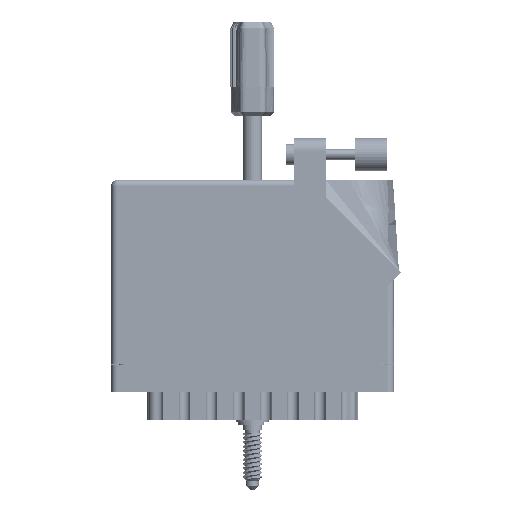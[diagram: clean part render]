
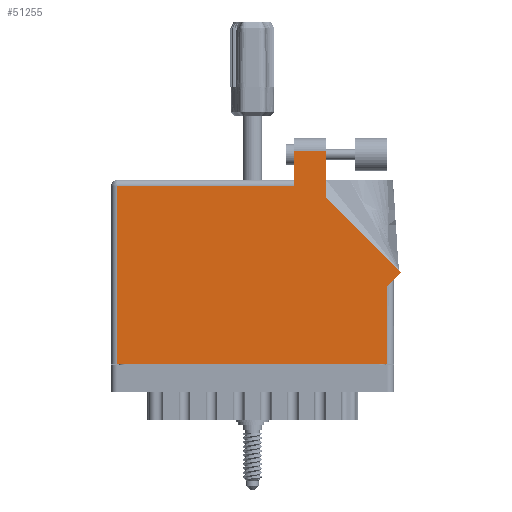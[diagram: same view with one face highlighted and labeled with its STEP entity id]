
A CAD part, front view. The second image highlights one B-rep face of the part: STEP entity #51255.
In plain terms, the highlighted face is planar.
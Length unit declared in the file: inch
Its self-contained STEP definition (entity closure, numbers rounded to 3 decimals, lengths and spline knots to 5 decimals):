
#1090 = CARTESIAN_POINT ( 'NONE',  ( 2.78871, 0.88571, 0. ) ) ;
#1462 = EDGE_LOOP ( 'NONE', ( #5592, #52478, #9378, #9748, #86802, #61947, #65933, #56642, #20698 ) ) ;
#2044 = VERTEX_POINT ( 'NONE', #49506 ) ;
#2688 = VECTOR ( 'NONE', #86116, 39.37008 ) ;
#2702 = VERTEX_POINT ( 'NONE', #65997 ) ;
#4891 = EDGE_CURVE ( 'NONE', #74700, #8188, #89115, .T. ) ;
#5466 = LINE ( 'NONE', #1090, #11969 ) ;
#5592 = ORIENTED_EDGE ( 'NONE', *, *, #35585, .T. ) ;
#8188 = VERTEX_POINT ( 'NONE', #80607 ) ;
#8299 = DIRECTION ( 'NONE',  ( 1., 0., 0. ) ) ;
#9378 = ORIENTED_EDGE ( 'NONE', *, *, #84445, .T. ) ;
#9748 = ORIENTED_EDGE ( 'NONE', *, *, #67827, .T. ) ;
#10830 = LINE ( 'NONE', #27716, #68132 ) ;
#11715 = LINE ( 'NONE', #42599, #64557 ) ;
#11969 = VECTOR ( 'NONE', #21018, 39.37008 ) ;
#13699 = VECTOR ( 'NONE', #65499, 39.37008 ) ;
#14456 = AXIS2_PLACEMENT_3D ( 'NONE', #31385, #65190, #31088 ) ;
#14808 = VERTEX_POINT ( 'NONE', #55230 ) ;
#16575 = VERTEX_POINT ( 'NONE', #45492 ) ;
#18417 = CARTESIAN_POINT ( 'NONE',  ( 0.062, 0., 0. ) ) ;
#20063 = DIRECTION ( 'NONE',  ( 0., -1., 0. ) ) ;
#20093 = LINE ( 'NONE', #28644, #50294 ) ;
#20698 = ORIENTED_EDGE ( 'NONE', *, *, #76182, .T. ) ;
#21018 = DIRECTION ( 'NONE',  ( -0.707, 0.707, 0. ) ) ;
#21892 = EDGE_CURVE ( 'NONE', #16575, #2044, #10830, .T. ) ;
#23826 = VERTEX_POINT ( 'NONE', #18417 ) ;
#24028 = VECTOR ( 'NONE', #76568, 39.37008 ) ;
#27570 = CARTESIAN_POINT ( 'NONE',  ( 0.062, 0., 0. ) ) ;
#27716 = CARTESIAN_POINT ( 'NONE',  ( 1.758, 2.05, 0. ) ) ;
#28562 = CARTESIAN_POINT ( 'NONE',  ( 2.656, 0.815, 0. ) ) ;
#28644 = CARTESIAN_POINT ( 'NONE',  ( 1.758, 1.775, 0. ) ) ;
#29662 = CARTESIAN_POINT ( 'NONE',  ( 1.758, 1.713, 0. ) ) ;
#30886 = CARTESIAN_POINT ( 'NONE',  ( 2.718, 0.815, 0. ) ) ;
#31086 = VECTOR ( 'NONE', #43551, 39.37008 ) ;
#31088 = DIRECTION ( 'NONE',  ( -1., 0., 0. ) ) ;
#31385 = CARTESIAN_POINT ( 'NONE',  ( 0., 1.775, 0. ) ) ;
#34385 = LINE ( 'NONE', #71325, #31086 ) ;
#35585 = EDGE_CURVE ( 'NONE', #2702, #16575, #34385, .T. ) ;
#35594 = DIRECTION ( 'NONE',  ( 0., -1., 0. ) ) ;
#38785 = EDGE_CURVE ( 'NONE', #81692, #74700, #75970, .T. ) ;
#42599 = CARTESIAN_POINT ( 'NONE',  ( 0., 0., 0. ) ) ;
#43551 = DIRECTION ( 'NONE',  ( 0., 1., 0. ) ) ;
#43863 = EDGE_CURVE ( 'NONE', #14808, #23826, #67130, .T. ) ;
#45492 = CARTESIAN_POINT ( 'NONE',  ( 2.065, 2.05, 0. ) ) ;
#49506 = CARTESIAN_POINT ( 'NONE',  ( 1.758, 2.05, 0. ) ) ;
#50294 = VECTOR ( 'NONE', #35594, 39.37008 ) ;
#51255 = ADVANCED_FACE ( 'NONE', ( #58485 ), #66387, .F. ) ;
#52478 = ORIENTED_EDGE ( 'NONE', *, *, #21892, .T. ) ;
#55230 = CARTESIAN_POINT ( 'NONE',  ( 0.062, 1.713, 0. ) ) ;
#56642 = ORIENTED_EDGE ( 'NONE', *, *, #4891, .T. ) ;
#58485 = FACE_OUTER_BOUND ( 'NONE', #1462, .T. ) ;
#61947 = ORIENTED_EDGE ( 'NONE', *, *, #80744, .T. ) ;
#64557 = VECTOR ( 'NONE', #8299, 39.37008 ) ;
#65190 = DIRECTION ( 'NONE',  ( 0., 0., -1. ) ) ;
#65342 = CARTESIAN_POINT ( 'NONE',  ( 2.656, 0.753, 0. ) ) ;
#65499 = DIRECTION ( 'NONE',  ( -1., 0., 0. ) ) ;
#65933 = ORIENTED_EDGE ( 'NONE', *, *, #38785, .T. ) ;
#65997 = CARTESIAN_POINT ( 'NONE',  ( 2.065, 1.60942, 0. ) ) ;
#66387 = PLANE ( 'NONE',  #14456 ) ;
#67130 = LINE ( 'NONE', #27570, #71451 ) ;
#67827 = EDGE_CURVE ( 'NONE', #83873, #14808, #71938, .T. ) ;
#68132 = VECTOR ( 'NONE', #89050, 39.37008 ) ;
#71325 = CARTESIAN_POINT ( 'NONE',  ( 2.065, 1.60942, 0. ) ) ;
#71451 = VECTOR ( 'NONE', #20063, 39.37008 ) ;
#71938 = LINE ( 'NONE', #77888, #13699 ) ;
#74700 = VERTEX_POINT ( 'NONE', #65342 ) ;
#75970 = LINE ( 'NONE', #28562, #24028 ) ;
#76182 = EDGE_CURVE ( 'NONE', #8188, #2702, #5466, .T. ) ;
#76568 = DIRECTION ( 'NONE',  ( 0., 1., 0. ) ) ;
#77888 = CARTESIAN_POINT ( 'NONE',  ( 0., 1.713, 0. ) ) ;
#80607 = CARTESIAN_POINT ( 'NONE',  ( 2.78871, 0.88571, 0. ) ) ;
#80744 = EDGE_CURVE ( 'NONE', #23826, #81692, #11715, .T. ) ;
#81692 = VERTEX_POINT ( 'NONE', #88057 ) ;
#83873 = VERTEX_POINT ( 'NONE', #29662 ) ;
#84445 = EDGE_CURVE ( 'NONE', #2044, #83873, #20093, .T. ) ;
#86116 = DIRECTION ( 'NONE',  ( 0.707, 0.707, 0. ) ) ;
#86802 = ORIENTED_EDGE ( 'NONE', *, *, #43863, .T. ) ;
#88057 = CARTESIAN_POINT ( 'NONE',  ( 2.656, 0., 0. ) ) ;
#89050 = DIRECTION ( 'NONE',  ( -1., 0., 0. ) ) ;
#89115 = LINE ( 'NONE', #30886, #2688 ) ;
